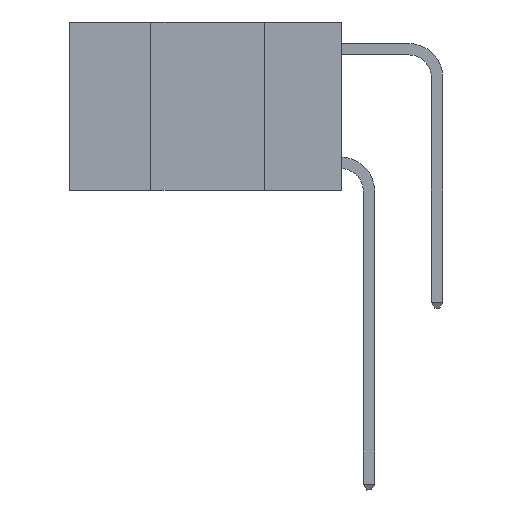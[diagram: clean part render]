
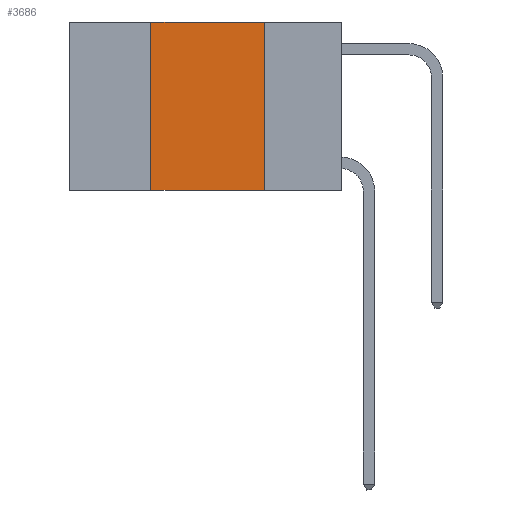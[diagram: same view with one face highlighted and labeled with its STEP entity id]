
A CAD part, left-side view. The second image highlights one B-rep face of the part: STEP entity #3686.
In plain terms, the highlighted planar face has unit normal (-1, 0, 0).
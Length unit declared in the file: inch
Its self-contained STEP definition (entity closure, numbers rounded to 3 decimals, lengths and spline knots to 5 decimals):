
#603 = VERTEX_POINT ( 'NONE', #11463 ) ;
#857 = LINE ( 'NONE', #10645, #1563 ) ;
#1563 = VECTOR ( 'NONE', #23698, 39.37008 ) ;
#2688 = PLANE ( 'NONE',  #27465 ) ;
#3241 = LINE ( 'NONE', #17186, #13499 ) ;
#3447 = EDGE_CURVE ( 'NONE', #11958, #603, #3241, .T. ) ;
#3686 = ADVANCED_FACE ( 'NONE', ( #11784 ), #2688, .F. ) ;
#5877 = EDGE_CURVE ( 'NONE', #13709, #603, #12330, .T. ) ;
#6574 = VECTOR ( 'NONE', #8392, 39.37008 ) ;
#6718 = CARTESIAN_POINT ( 'NONE',  ( 0., 0.42, 0. ) ) ;
#7168 = DIRECTION ( 'NONE',  ( 0., 0., -1. ) ) ;
#7873 = EDGE_CURVE ( 'NONE', #11958, #14703, #15299, .T. ) ;
#8293 = CARTESIAN_POINT ( 'NONE',  ( 0., 0.42, 0. ) ) ;
#8392 = DIRECTION ( 'NONE',  ( 0., 0., -1. ) ) ;
#8409 = DIRECTION ( 'NONE',  ( 0., -1., 0. ) ) ;
#8859 = ORIENTED_EDGE ( 'NONE', *, *, #3447, .T. ) ;
#10194 = VECTOR ( 'NONE', #10490, 39.37008 ) ;
#10490 = DIRECTION ( 'NONE',  ( 0., 0., 1. ) ) ;
#10645 = CARTESIAN_POINT ( 'NONE',  ( 0., 0.6, 0. ) ) ;
#11463 = CARTESIAN_POINT ( 'NONE',  ( 0., 0.17, -0.37 ) ) ;
#11784 = FACE_OUTER_BOUND ( 'NONE', #23370, .T. ) ;
#11958 = VERTEX_POINT ( 'NONE', #27533 ) ;
#12330 = LINE ( 'NONE', #25726, #6574 ) ;
#12552 = ORIENTED_EDGE ( 'NONE', *, *, #5877, .F. ) ;
#13499 = VECTOR ( 'NONE', #8409, 39.37008 ) ;
#13709 = VERTEX_POINT ( 'NONE', #20384 ) ;
#14703 = VERTEX_POINT ( 'NONE', #6718 ) ;
#15299 = LINE ( 'NONE', #8293, #10194 ) ;
#16035 = EDGE_CURVE ( 'NONE', #14703, #13709, #857, .T. ) ;
#16348 = ORIENTED_EDGE ( 'NONE', *, *, #7873, .F. ) ;
#17186 = CARTESIAN_POINT ( 'NONE',  ( 0., 0.6, -0.37 ) ) ;
#18022 = CARTESIAN_POINT ( 'NONE',  ( 0., 0.6, 0. ) ) ;
#20191 = DIRECTION ( 'NONE',  ( 1., 0., 0. ) ) ;
#20384 = CARTESIAN_POINT ( 'NONE',  ( 0., 0.17, 0. ) ) ;
#22431 = ORIENTED_EDGE ( 'NONE', *, *, #16035, .F. ) ;
#23370 = EDGE_LOOP ( 'NONE', ( #12552, #22431, #16348, #8859 ) ) ;
#23698 = DIRECTION ( 'NONE',  ( 0., -1., 0. ) ) ;
#25726 = CARTESIAN_POINT ( 'NONE',  ( 0., 0.17, 0. ) ) ;
#27465 = AXIS2_PLACEMENT_3D ( 'NONE', #18022, #20191, #7168 ) ;
#27533 = CARTESIAN_POINT ( 'NONE',  ( 0., 0.42, -0.37 ) ) ;
